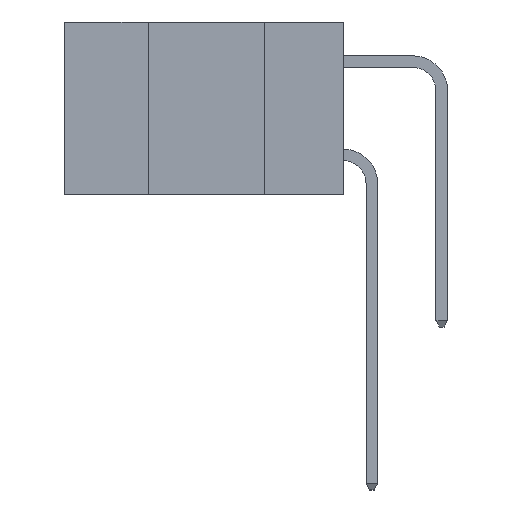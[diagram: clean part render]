
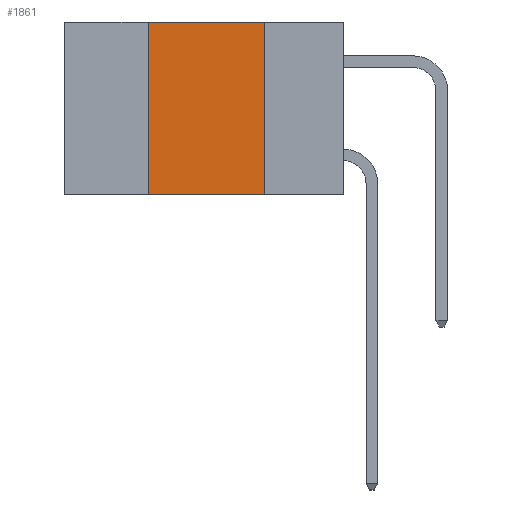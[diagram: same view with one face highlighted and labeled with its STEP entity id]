
A CAD part, left-side view. The second image highlights one B-rep face of the part: STEP entity #1861.
In plain terms, the highlighted planar face has unit normal (-1, 0, 0).
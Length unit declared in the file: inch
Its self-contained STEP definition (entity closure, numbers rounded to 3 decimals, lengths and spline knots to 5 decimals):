
#367 = LINE ( 'NONE', #11088, #5025 ) ;
#543 = DIRECTION ( 'NONE',  ( 0., -1., 0. ) ) ;
#888 = DIRECTION ( 'NONE',  ( 0., 0., -1. ) ) ;
#1528 = VERTEX_POINT ( 'NONE', #12298 ) ;
#1861 = ADVANCED_FACE ( 'NONE', ( #4404 ), #8868, .F. ) ;
#2295 = VECTOR ( 'NONE', #543, 39.37008 ) ;
#2467 = LINE ( 'NONE', #21845, #10925 ) ;
#2737 = EDGE_LOOP ( 'NONE', ( #12649, #9836, #9444, #20716 ) ) ;
#4360 = EDGE_CURVE ( 'NONE', #1528, #8471, #15119, .T. ) ;
#4404 = FACE_OUTER_BOUND ( 'NONE', #2737, .T. ) ;
#5025 = VECTOR ( 'NONE', #888, 39.37008 ) ;
#6815 = CARTESIAN_POINT ( 'NONE',  ( 0., 0.6, 0. ) ) ;
#6848 = LINE ( 'NONE', #20836, #2295 ) ;
#6854 = DIRECTION ( 'NONE',  ( 0., -1., 0. ) ) ;
#7633 = VERTEX_POINT ( 'NONE', #12731 ) ;
#8066 = DIRECTION ( 'NONE',  ( 0., 0., -1. ) ) ;
#8471 = VERTEX_POINT ( 'NONE', #18017 ) ;
#8523 = DIRECTION ( 'NONE',  ( 1., 0., 0. ) ) ;
#8814 = CARTESIAN_POINT ( 'NONE',  ( 0., 0.6, 0. ) ) ;
#8868 = PLANE ( 'NONE',  #12577 ) ;
#9444 = ORIENTED_EDGE ( 'NONE', *, *, #14821, .F. ) ;
#9836 = ORIENTED_EDGE ( 'NONE', *, *, #4360, .F. ) ;
#10925 = VECTOR ( 'NONE', #20243, 39.37008 ) ;
#11088 = CARTESIAN_POINT ( 'NONE',  ( 0., 0.17, -0.37 ) ) ;
#11227 = CARTESIAN_POINT ( 'NONE',  ( 0., 0.42, -0.37 ) ) ;
#12183 = EDGE_CURVE ( 'NONE', #8471, #7633, #367, .T. ) ;
#12298 = CARTESIAN_POINT ( 'NONE',  ( 0., 0.42, 0. ) ) ;
#12577 = AXIS2_PLACEMENT_3D ( 'NONE', #8814, #8523, #8066 ) ;
#12649 = ORIENTED_EDGE ( 'NONE', *, *, #12183, .F. ) ;
#12731 = CARTESIAN_POINT ( 'NONE',  ( 0., 0.17, -0.37 ) ) ;
#12784 = EDGE_CURVE ( 'NONE', #19662, #7633, #6848, .T. ) ;
#14821 = EDGE_CURVE ( 'NONE', #19662, #1528, #2467, .T. ) ;
#15119 = LINE ( 'NONE', #6815, #19647 ) ;
#18017 = CARTESIAN_POINT ( 'NONE',  ( 0., 0.17, 0. ) ) ;
#19647 = VECTOR ( 'NONE', #6854, 39.37008 ) ;
#19662 = VERTEX_POINT ( 'NONE', #11227 ) ;
#20243 = DIRECTION ( 'NONE',  ( 0., 0., 1. ) ) ;
#20716 = ORIENTED_EDGE ( 'NONE', *, *, #12784, .T. ) ;
#20836 = CARTESIAN_POINT ( 'NONE',  ( 0., 0.6, -0.37 ) ) ;
#21845 = CARTESIAN_POINT ( 'NONE',  ( 0., 0.42, -0.37 ) ) ;
